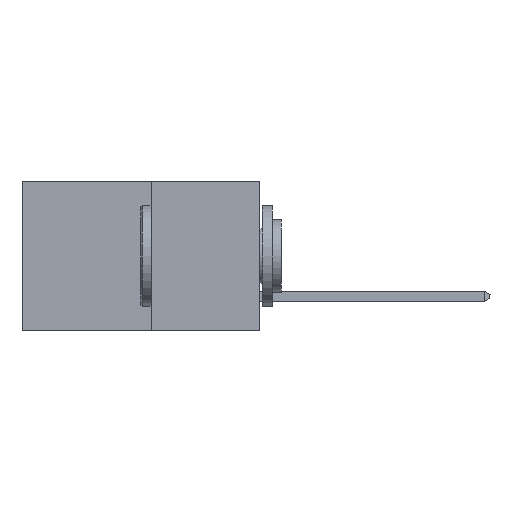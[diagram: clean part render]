
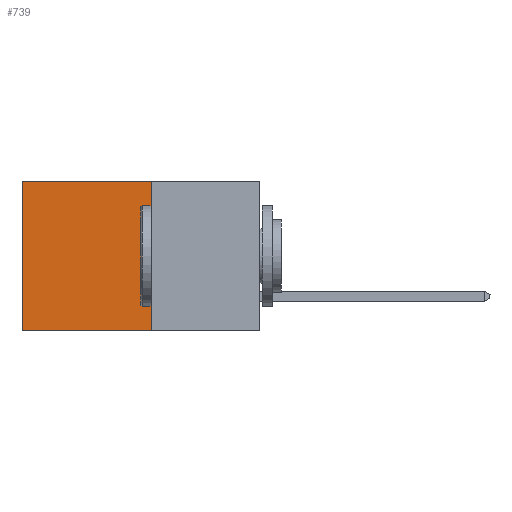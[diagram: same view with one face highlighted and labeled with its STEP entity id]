
A CAD part, left-side view. The second image highlights one B-rep face of the part: STEP entity #739.
In plain terms, the highlighted planar face has unit normal (-1, 0, 0).
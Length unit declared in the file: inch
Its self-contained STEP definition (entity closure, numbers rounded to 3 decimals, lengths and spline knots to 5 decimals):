
#594 = LINE ( 'NONE', #18730, #5204 ) ;
#739 = ADVANCED_FACE ( 'NONE', ( #2047 ), #14897, .F. ) ;
#2047 = FACE_OUTER_BOUND ( 'NONE', #2479, .T. ) ;
#2479 = EDGE_LOOP ( 'NONE', ( #17636, #6955, #3072, #18447 ) ) ;
#2991 = LINE ( 'NONE', #10375, #7572 ) ;
#3072 = ORIENTED_EDGE ( 'NONE', *, *, #18462, .F. ) ;
#5204 = VECTOR ( 'NONE', #20618, 39.37008 ) ;
#5638 = CARTESIAN_POINT ( 'NONE',  ( 0.277, 0.27, 0. ) ) ;
#5723 = AXIS2_PLACEMENT_3D ( 'NONE', #15161, #14843, #15798 ) ;
#6955 = ORIENTED_EDGE ( 'NONE', *, *, #22216, .F. ) ;
#7090 = LINE ( 'NONE', #18184, #11573 ) ;
#7567 = DIRECTION ( 'NONE',  ( 0., 1., 0. ) ) ;
#7572 = VECTOR ( 'NONE', #12283, 39.37008 ) ;
#8356 = VERTEX_POINT ( 'NONE', #23530 ) ;
#8571 = CARTESIAN_POINT ( 'NONE',  ( 0.277, 0.59, 0. ) ) ;
#9397 = LINE ( 'NONE', #5638, #18946 ) ;
#10375 = CARTESIAN_POINT ( 'NONE',  ( 0.277, 0.27, -0.37 ) ) ;
#10557 = EDGE_CURVE ( 'NONE', #12945, #8356, #7090, .T. ) ;
#11573 = VECTOR ( 'NONE', #14295, 39.37008 ) ;
#12283 = DIRECTION ( 'NONE',  ( 0., 1., 0. ) ) ;
#12581 = EDGE_CURVE ( 'NONE', #20377, #12945, #9397, .T. ) ;
#12945 = VERTEX_POINT ( 'NONE', #8571 ) ;
#14295 = DIRECTION ( 'NONE',  ( 0., 0., -1. ) ) ;
#14843 = DIRECTION ( 'NONE',  ( 1., 0., 0. ) ) ;
#14897 = PLANE ( 'NONE',  #5723 ) ;
#15161 = CARTESIAN_POINT ( 'NONE',  ( 0.277, 0.27, -0.37 ) ) ;
#15798 = DIRECTION ( 'NONE',  ( 0., 0., -1. ) ) ;
#16649 = CARTESIAN_POINT ( 'NONE',  ( 0.277, 0.27, 0. ) ) ;
#17636 = ORIENTED_EDGE ( 'NONE', *, *, #10557, .T. ) ;
#18184 = CARTESIAN_POINT ( 'NONE',  ( 0.277, 0.59, -0.37 ) ) ;
#18447 = ORIENTED_EDGE ( 'NONE', *, *, #12581, .T. ) ;
#18462 = EDGE_CURVE ( 'NONE', #20377, #18725, #594, .T. ) ;
#18725 = VERTEX_POINT ( 'NONE', #23233 ) ;
#18730 = CARTESIAN_POINT ( 'NONE',  ( 0.277, 0.27, -0.37 ) ) ;
#18946 = VECTOR ( 'NONE', #7567, 39.37008 ) ;
#20377 = VERTEX_POINT ( 'NONE', #16649 ) ;
#20618 = DIRECTION ( 'NONE',  ( 0., 0., -1. ) ) ;
#22216 = EDGE_CURVE ( 'NONE', #18725, #8356, #2991, .T. ) ;
#23233 = CARTESIAN_POINT ( 'NONE',  ( 0.277, 0.27, -0.37 ) ) ;
#23530 = CARTESIAN_POINT ( 'NONE',  ( 0.277, 0.59, -0.37 ) ) ;
